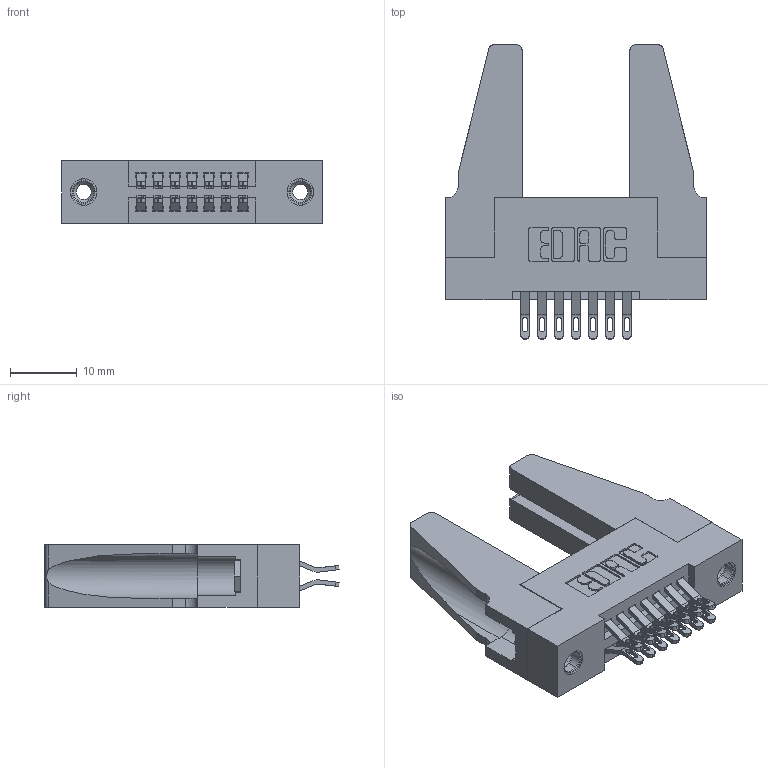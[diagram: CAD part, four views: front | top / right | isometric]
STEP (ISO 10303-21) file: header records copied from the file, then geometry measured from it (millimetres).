
FILE_DESCRIPTION (( 'STEP AP203' ), '1' );
FILE_NAME ('395-014-555-288.STEP', '2019-10-15T16:38:19', ( '' ), ( '' ), 'SwSTEP 2.0', 'SolidWorks 2016', '' );
FILE_SCHEMA (( 'CONFIG_CONTROL_DESIGN' ));
Length unit declared in the file: inch
Products named in the file (5): 345-220-078_345-220-088; 395-014-555-288; 345 Part_Flush Mounting Lugs - 0.156 Dia-TH; 345-292-001_555 Tail; 345-250-001_345-250-001-102
Assembly tree (19 placements, depth 2):
  395-014-555-288
    345 Part_Flush Mounting Lugs - 0.156 Dia-TH
    345-292-001_555 Tail  x14
    345-250-001_345-250-001-102  x2
    345-220-078_345-220-088  x2
Bounding box: 39.01 x 43.99 x 9.4 mm (x, y, z)
Volume: 6758.1 mm3; surface area: 7767.4 mm2
Topology: 19 solids, 19 shells, 1034 faces, 3133 edges, 2078 vertices
Faces by surface type: plane 586, cylinder 432, cone 12, torus 4
Entity records: 12678 total; most frequent: CARTESIAN_POINT 2188, ORIENTED_EDGE 2052, DIRECTION 1946, EDGE_CURVE 1026, LINE 804, VECTOR 804, VERTEX_POINT 678, AXIS2_PLACEMENT_3D 571
